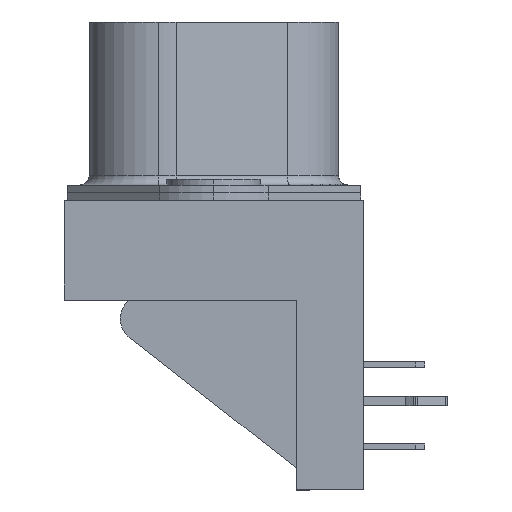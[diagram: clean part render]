
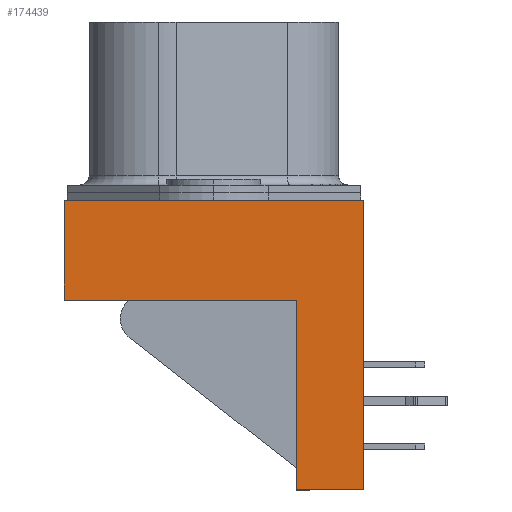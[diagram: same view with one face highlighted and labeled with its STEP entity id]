
A CAD part, left-side view. The second image highlights one B-rep face of the part: STEP entity #174439.
In plain terms, the highlighted planar face has unit normal (-1, 0, 0).
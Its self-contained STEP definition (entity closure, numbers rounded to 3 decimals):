
#940 = DIRECTION ( 'NONE',  ( 0., -1., 0. ) ) ;
#7701 = LINE ( 'NONE', #63292, #161716 ) ;
#14744 = ORIENTED_EDGE ( 'NONE', *, *, #123465, .F. ) ;
#17133 = EDGE_CURVE ( 'NONE', #35204, #116085, #106666, .T. ) ;
#18782 = CARTESIAN_POINT ( 'NONE',  ( -4.125, 7.8, 0. ) ) ;
#18929 = CARTESIAN_POINT ( 'NONE',  ( -4.125, -7.8, 0. ) ) ;
#21711 = AXIS2_PLACEMENT_3D ( 'NONE', #62665, #90417, #158490 ) ;
#25136 = DIRECTION ( 'NONE',  ( 0., 0., 1. ) ) ;
#26018 = ORIENTED_EDGE ( 'NONE', *, *, #60773, .F. ) ;
#35204 = VERTEX_POINT ( 'NONE', #124281 ) ;
#35463 = EDGE_CURVE ( 'NONE', #39568, #35204, #7701, .T. ) ;
#39568 = VERTEX_POINT ( 'NONE', #117049 ) ;
#43649 = ORIENTED_EDGE ( 'NONE', *, *, #35463, .T. ) ;
#49208 = FACE_OUTER_BOUND ( 'NONE', #101299, .T. ) ;
#50852 = EDGE_CURVE ( 'NONE', #39568, #54836, #106727, .T. ) ;
#54836 = VERTEX_POINT ( 'NONE', #132716 ) ;
#60709 = CARTESIAN_POINT ( 'NONE',  ( -4.125, 7.8, 0. ) ) ;
#60773 = EDGE_CURVE ( 'NONE', #157659, #116085, #141523, .T. ) ;
#62665 = CARTESIAN_POINT ( 'NONE',  ( -4.125, 7.8, -15.1 ) ) ;
#63292 = CARTESIAN_POINT ( 'NONE',  ( -4.125, 7.8, -15.1 ) ) ;
#63760 = VERTEX_POINT ( 'NONE', #142241 ) ;
#64712 = CARTESIAN_POINT ( 'NONE',  ( -4.125, -4.3, -15.1 ) ) ;
#75313 = VECTOR ( 'NONE', #151752, 1000. ) ;
#78523 = VECTOR ( 'NONE', #97328, 1000. ) ;
#81600 = CARTESIAN_POINT ( 'NONE',  ( -4.125, -7.8, -15.1 ) ) ;
#90153 = DIRECTION ( 'NONE',  ( 0., -1., 0. ) ) ;
#90417 = DIRECTION ( 'NONE',  ( -1., 0., 0. ) ) ;
#94069 = ORIENTED_EDGE ( 'NONE', *, *, #17133, .T. ) ;
#97120 = CARTESIAN_POINT ( 'NONE',  ( -4.125, 7.8, -5.2 ) ) ;
#97328 = DIRECTION ( 'NONE',  ( 0., 0., 1. ) ) ;
#98776 = ORIENTED_EDGE ( 'NONE', *, *, #50852, .F. ) ;
#101299 = EDGE_LOOP ( 'NONE', ( #14744, #98776, #43649, #94069, #26018, #155963 ) ) ;
#106666 = LINE ( 'NONE', #81600, #140394 ) ;
#106727 = LINE ( 'NONE', #64712, #108566 ) ;
#107354 = PLANE ( 'NONE',  #21711 ) ;
#108566 = VECTOR ( 'NONE', #120188, 1000. ) ;
#116085 = VERTEX_POINT ( 'NONE', #18929 ) ;
#117049 = CARTESIAN_POINT ( 'NONE',  ( -4.125, -4.3, -15.1 ) ) ;
#120188 = DIRECTION ( 'NONE',  ( 0., 0., 1. ) ) ;
#123465 = EDGE_CURVE ( 'NONE', #54836, #63760, #123991, .T. ) ;
#123991 = LINE ( 'NONE', #97120, #75313 ) ;
#124196 = LINE ( 'NONE', #154611, #78523 ) ;
#124281 = CARTESIAN_POINT ( 'NONE',  ( -4.125, -7.8, -15.1 ) ) ;
#132716 = CARTESIAN_POINT ( 'NONE',  ( -4.125, -4.3, -5.2 ) ) ;
#140394 = VECTOR ( 'NONE', #25136, 1000. ) ;
#141523 = LINE ( 'NONE', #18782, #164269 ) ;
#142241 = CARTESIAN_POINT ( 'NONE',  ( -4.125, 7.8, -5.2 ) ) ;
#151752 = DIRECTION ( 'NONE',  ( 0., 1., 0. ) ) ;
#154611 = CARTESIAN_POINT ( 'NONE',  ( -4.125, 7.8, -15.1 ) ) ;
#155369 = EDGE_CURVE ( 'NONE', #63760, #157659, #124196, .T. ) ;
#155963 = ORIENTED_EDGE ( 'NONE', *, *, #155369, .F. ) ;
#157659 = VERTEX_POINT ( 'NONE', #60709 ) ;
#158490 = DIRECTION ( 'NONE',  ( 0., -1., 0. ) ) ;
#161716 = VECTOR ( 'NONE', #90153, 1000. ) ;
#164269 = VECTOR ( 'NONE', #940, 1000. ) ;
#174439 = ADVANCED_FACE ( 'NONE', ( #49208 ), #107354, .T. ) ;
